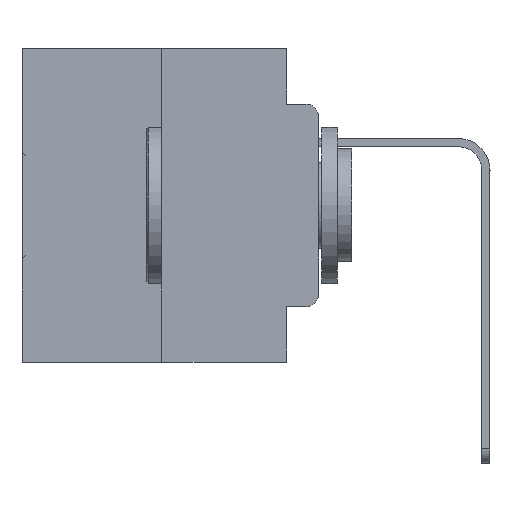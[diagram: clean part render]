
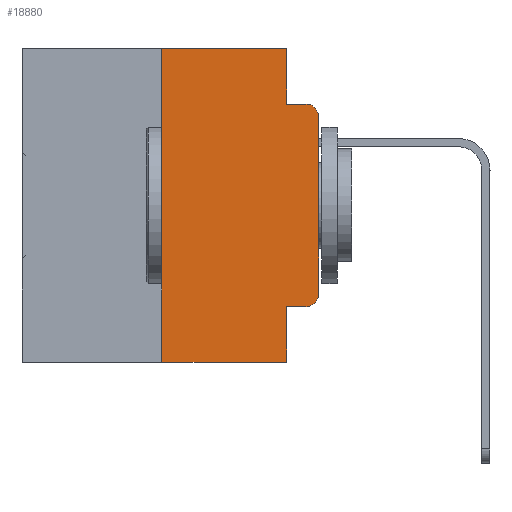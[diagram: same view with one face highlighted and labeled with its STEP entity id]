
A CAD part, left-side view. The second image highlights one B-rep face of the part: STEP entity #18880.
In plain terms, the highlighted planar face has unit normal (-1, 0, 0).
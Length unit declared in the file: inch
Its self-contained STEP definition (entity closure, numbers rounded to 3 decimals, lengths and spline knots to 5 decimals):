
#230 = CARTESIAN_POINT ( 'NONE',  ( 0., 0.473, 0. ) ) ;
#531 = VERTEX_POINT ( 'NONE', #13448 ) ;
#565 = CARTESIAN_POINT ( 'NONE',  ( 0., 0.051, 0. ) ) ;
#670 = VECTOR ( 'NONE', #31915, 39.37008 ) ;
#1208 = VECTOR ( 'NONE', #13433, 39.37008 ) ;
#1845 = ORIENTED_EDGE ( 'NONE', *, *, #15828, .T. ) ;
#2684 = ORIENTED_EDGE ( 'NONE', *, *, #19321, .T. ) ;
#2718 = CARTESIAN_POINT ( 'NONE',  ( 0., 0.25, 0. ) ) ;
#2726 = AXIS2_PLACEMENT_3D ( 'NONE', #29917, #7329, #14689 ) ;
#2824 = EDGE_CURVE ( 'NONE', #14557, #531, #3834, .T. ) ;
#2856 = DIRECTION ( 'NONE',  ( 0., -1., 0. ) ) ;
#3834 = LINE ( 'NONE', #2718, #31249 ) ;
#4129 = VECTOR ( 'NONE', #20043, 39.37008 ) ;
#5050 = CARTESIAN_POINT ( 'NONE',  ( 0., 0.02, -0.1085 ) ) ;
#5075 = EDGE_LOOP ( 'NONE', ( #20645, #1845, #29588, #9398, #16294, #26829, #2684, #21751, #22606, #15434 ) ) ;
#5620 = CARTESIAN_POINT ( 'NONE',  ( 0., 0., 0. ) ) ;
#6447 = VECTOR ( 'NONE', #25936, 39.37008 ) ;
#7305 = EDGE_CURVE ( 'NONE', #531, #11743, #10680, .T. ) ;
#7329 = DIRECTION ( 'NONE',  ( 1., 0., 0. ) ) ;
#7396 = DIRECTION ( 'NONE',  ( -1., 0., 0. ) ) ;
#8024 = CARTESIAN_POINT ( 'NONE',  ( 0., 0.051, -0.4115 ) ) ;
#8056 = EDGE_CURVE ( 'NONE', #8672, #27147, #11032, .T. ) ;
#8096 = EDGE_CURVE ( 'NONE', #19760, #15581, #8691, .T. ) ;
#8543 = VECTOR ( 'NONE', #2856, 39.37008 ) ;
#8672 = VERTEX_POINT ( 'NONE', #16952 ) ;
#8691 = CIRCLE ( 'NONE', #26560, 0.02 ) ;
#9398 = ORIENTED_EDGE ( 'NONE', *, *, #28715, .F. ) ;
#10680 = LINE ( 'NONE', #230, #4129 ) ;
#11017 = CARTESIAN_POINT ( 'NONE',  ( 0., 0.473, -0.5 ) ) ;
#11032 = LINE ( 'NONE', #19277, #31502 ) ;
#11155 = EDGE_CURVE ( 'NONE', #13503, #25353, #16957, .T. ) ;
#11743 = VERTEX_POINT ( 'NONE', #565 ) ;
#12703 = DIRECTION ( 'NONE',  ( 0., 0., -1. ) ) ;
#12722 = CARTESIAN_POINT ( 'NONE',  ( 0., 0.02, -0.4115 ) ) ;
#13433 = DIRECTION ( 'NONE',  ( 0., 0., -1. ) ) ;
#13448 = CARTESIAN_POINT ( 'NONE',  ( 0., 0.25, 0. ) ) ;
#13503 = VERTEX_POINT ( 'NONE', #21860 ) ;
#13662 = FACE_OUTER_BOUND ( 'NONE', #5075, .T. ) ;
#14293 = LINE ( 'NONE', #5620, #21630 ) ;
#14356 = LINE ( 'NONE', #23506, #1208 ) ;
#14557 = VERTEX_POINT ( 'NONE', #30211 ) ;
#14689 = DIRECTION ( 'NONE',  ( 0., 0., -1. ) ) ;
#15226 = VERTEX_POINT ( 'NONE', #19683 ) ;
#15418 = EDGE_CURVE ( 'NONE', #15581, #15226, #14293, .T. ) ;
#15434 = ORIENTED_EDGE ( 'NONE', *, *, #8096, .T. ) ;
#15581 = VERTEX_POINT ( 'NONE', #16408 ) ;
#15828 = EDGE_CURVE ( 'NONE', #15226, #27147, #25704, .T. ) ;
#15877 = CARTESIAN_POINT ( 'NONE',  ( 0., 0.02, -0.0885 ) ) ;
#16294 = ORIENTED_EDGE ( 'NONE', *, *, #7305, .F. ) ;
#16408 = CARTESIAN_POINT ( 'NONE',  ( 0., 0., -0.3915 ) ) ;
#16952 = CARTESIAN_POINT ( 'NONE',  ( 0., 0.051, -0.0885 ) ) ;
#16957 = LINE ( 'NONE', #19334, #670 ) ;
#18880 = ADVANCED_FACE ( 'NONE', ( #13662 ), #27121, .F. ) ;
#19277 = CARTESIAN_POINT ( 'NONE',  ( 0., 0.051, -0.0885 ) ) ;
#19321 = EDGE_CURVE ( 'NONE', #14557, #25353, #25012, .T. ) ;
#19334 = CARTESIAN_POINT ( 'NONE',  ( 0., 0.051, 0. ) ) ;
#19683 = CARTESIAN_POINT ( 'NONE',  ( 0., 0., -0.1085 ) ) ;
#19760 = VERTEX_POINT ( 'NONE', #12722 ) ;
#20027 = DIRECTION ( 'NONE',  ( 0., 0., 1. ) ) ;
#20043 = DIRECTION ( 'NONE',  ( 0., -1., 0. ) ) ;
#20645 = ORIENTED_EDGE ( 'NONE', *, *, #15418, .T. ) ;
#21630 = VECTOR ( 'NONE', #28399, 39.37008 ) ;
#21751 = ORIENTED_EDGE ( 'NONE', *, *, #11155, .F. ) ;
#21860 = CARTESIAN_POINT ( 'NONE',  ( 0., 0.051, -0.4115 ) ) ;
#22480 = DIRECTION ( 'NONE',  ( -1., 0., 0. ) ) ;
#22606 = ORIENTED_EDGE ( 'NONE', *, *, #28604, .T. ) ;
#23506 = CARTESIAN_POINT ( 'NONE',  ( 0., 0.051, 0. ) ) ;
#24617 = AXIS2_PLACEMENT_3D ( 'NONE', #5050, #7396, #12703 ) ;
#25012 = LINE ( 'NONE', #11017, #6447 ) ;
#25353 = VERTEX_POINT ( 'NONE', #25940 ) ;
#25704 = CIRCLE ( 'NONE', #24617, 0.02 ) ;
#25936 = DIRECTION ( 'NONE',  ( 0., -1., 0. ) ) ;
#25940 = CARTESIAN_POINT ( 'NONE',  ( 0., 0.051, -0.5 ) ) ;
#26560 = AXIS2_PLACEMENT_3D ( 'NONE', #29809, #22480, #29704 ) ;
#26829 = ORIENTED_EDGE ( 'NONE', *, *, #2824, .F. ) ;
#27121 = PLANE ( 'NONE',  #2726 ) ;
#27147 = VERTEX_POINT ( 'NONE', #15877 ) ;
#28399 = DIRECTION ( 'NONE',  ( 0., 0., 1. ) ) ;
#28604 = EDGE_CURVE ( 'NONE', #13503, #19760, #31740, .T. ) ;
#28715 = EDGE_CURVE ( 'NONE', #11743, #8672, #14356, .T. ) ;
#29285 = DIRECTION ( 'NONE',  ( 0., -1., 0. ) ) ;
#29588 = ORIENTED_EDGE ( 'NONE', *, *, #8056, .F. ) ;
#29704 = DIRECTION ( 'NONE',  ( 0., 0., -1. ) ) ;
#29809 = CARTESIAN_POINT ( 'NONE',  ( 0., 0.02, -0.3915 ) ) ;
#29917 = CARTESIAN_POINT ( 'NONE',  ( 0., 0.473, 0. ) ) ;
#30211 = CARTESIAN_POINT ( 'NONE',  ( 0., 0.25, -0.5 ) ) ;
#31249 = VECTOR ( 'NONE', #20027, 39.37008 ) ;
#31502 = VECTOR ( 'NONE', #29285, 39.37008 ) ;
#31740 = LINE ( 'NONE', #8024, #8543 ) ;
#31915 = DIRECTION ( 'NONE',  ( 0., 0., -1. ) ) ;
